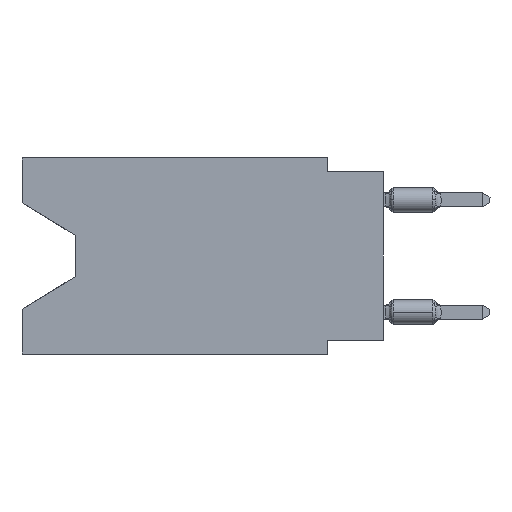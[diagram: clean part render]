
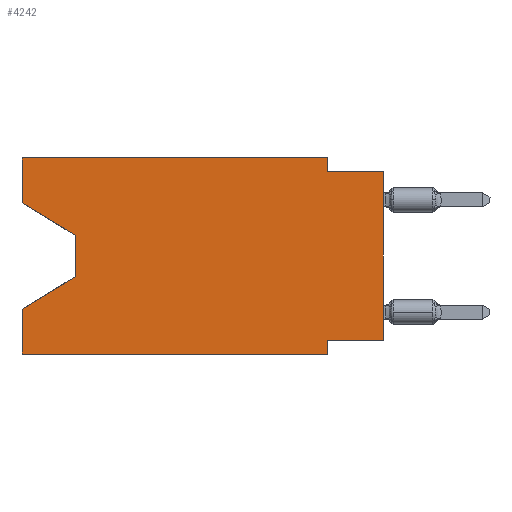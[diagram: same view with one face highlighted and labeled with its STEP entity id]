
A CAD part, left-side view. The second image highlights one B-rep face of the part: STEP entity #4242.
In plain terms, the highlighted planar face has unit normal (-1, 0, 0).
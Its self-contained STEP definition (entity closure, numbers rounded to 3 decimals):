
#185 = VECTOR ( 'NONE', #11894, 1000. ) ;
#356 = LINE ( 'NONE', #1703, #1404 ) ;
#411 = ORIENTED_EDGE ( 'NONE', *, *, #1171, .T. ) ;
#521 = CARTESIAN_POINT ( 'NONE',  ( 0., 16.383, -6.852 ) ) ;
#795 = ORIENTED_EDGE ( 'NONE', *, *, #1060, .F. ) ;
#810 = EDGE_CURVE ( 'NONE', #8249, #14332, #7333, .T. ) ;
#878 = DIRECTION ( 'NONE',  ( 0., 1., 0. ) ) ;
#1060 = EDGE_CURVE ( 'NONE', #10597, #8249, #9321, .T. ) ;
#1171 = EDGE_CURVE ( 'NONE', #6438, #5531, #4369, .T. ) ;
#1404 = VECTOR ( 'NONE', #15974, 1000. ) ;
#1484 = DIRECTION ( 'NONE',  ( 0., 0., 1. ) ) ;
#1649 = VECTOR ( 'NONE', #13506, 1000. ) ;
#1703 = CARTESIAN_POINT ( 'NONE',  ( 0., 16.383, 0. ) ) ;
#1808 = ORIENTED_EDGE ( 'NONE', *, *, #6206, .T. ) ;
#1897 = ORIENTED_EDGE ( 'NONE', *, *, #810, .F. ) ;
#1899 = EDGE_CURVE ( 'NONE', #4299, #14967, #3849, .T. ) ;
#2055 = DIRECTION ( 'NONE',  ( 0., 0., -1. ) ) ;
#2230 = ORIENTED_EDGE ( 'NONE', *, *, #13878, .F. ) ;
#2676 = CARTESIAN_POINT ( 'NONE',  ( 0., 0., 0. ) ) ;
#2705 = VECTOR ( 'NONE', #11100, 1000. ) ;
#2866 = DIRECTION ( 'NONE',  ( 0., -0.855, -0.519 ) ) ;
#3119 = DIRECTION ( 'NONE',  ( 0., 0.855, -0.519 ) ) ;
#3222 = LINE ( 'NONE', #3475, #2705 ) ;
#3268 = CARTESIAN_POINT ( 'NONE',  ( 0., 0., -0.635 ) ) ;
#3475 = CARTESIAN_POINT ( 'NONE',  ( 0., 13.97, -3.505 ) ) ;
#3585 = LINE ( 'NONE', #13564, #7026 ) ;
#3849 = LINE ( 'NONE', #15668, #185 ) ;
#4203 = CARTESIAN_POINT ( 'NONE',  ( 0., 16.383, -2.038 ) ) ;
#4235 = CARTESIAN_POINT ( 'NONE',  ( 0., 0., -0.635 ) ) ;
#4242 = ADVANCED_FACE ( 'NONE', ( #8076 ), #5472, .F. ) ;
#4299 = VERTEX_POINT ( 'NONE', #13042 ) ;
#4369 = LINE ( 'NONE', #12342, #7140 ) ;
#4659 = LINE ( 'NONE', #15152, #6732 ) ;
#4800 = EDGE_LOOP ( 'NONE', ( #8580, #10846, #411, #11090, #5326, #16095, #9362, #1808, #2230, #9218, #1897, #795 ) ) ;
#5311 = CARTESIAN_POINT ( 'NONE',  ( 0., 16.383, 0. ) ) ;
#5326 = ORIENTED_EDGE ( 'NONE', *, *, #11420, .T. ) ;
#5329 = CARTESIAN_POINT ( 'NONE',  ( 0., 16.383, -8.89 ) ) ;
#5387 = DIRECTION ( 'NONE',  ( 0., 0., 1. ) ) ;
#5408 = LINE ( 'NONE', #5329, #12397 ) ;
#5472 = PLANE ( 'NONE',  #11635 ) ;
#5508 = VERTEX_POINT ( 'NONE', #4235 ) ;
#5531 = VERTEX_POINT ( 'NONE', #521 ) ;
#5663 = EDGE_CURVE ( 'NONE', #11098, #6438, #3222, .T. ) ;
#6206 = EDGE_CURVE ( 'NONE', #13308, #5508, #6693, .T. ) ;
#6412 = EDGE_CURVE ( 'NONE', #13308, #4299, #4659, .T. ) ;
#6438 = VERTEX_POINT ( 'NONE', #13908 ) ;
#6693 = LINE ( 'NONE', #2676, #12910 ) ;
#6732 = VECTOR ( 'NONE', #878, 1000. ) ;
#6855 = VECTOR ( 'NONE', #9663, 1000. ) ;
#7026 = VECTOR ( 'NONE', #2055, 1000. ) ;
#7140 = VECTOR ( 'NONE', #3119, 1000. ) ;
#7333 = LINE ( 'NONE', #12450, #6855 ) ;
#7407 = VECTOR ( 'NONE', #2866, 1000. ) ;
#7524 = CARTESIAN_POINT ( 'NONE',  ( 0., 2.54, 0. ) ) ;
#8026 = CARTESIAN_POINT ( 'NONE',  ( 0., 13.97, -3.505 ) ) ;
#8076 = FACE_OUTER_BOUND ( 'NONE', #4800, .T. ) ;
#8249 = VERTEX_POINT ( 'NONE', #13566 ) ;
#8580 = ORIENTED_EDGE ( 'NONE', *, *, #10630, .T. ) ;
#9093 = DIRECTION ( 'NONE',  ( 0., 0., -1. ) ) ;
#9200 = VERTEX_POINT ( 'NONE', #12933 ) ;
#9218 = ORIENTED_EDGE ( 'NONE', *, *, #14282, .F. ) ;
#9241 = CARTESIAN_POINT ( 'NONE',  ( 0., 16.383, 0. ) ) ;
#9321 = LINE ( 'NONE', #5311, #15992 ) ;
#9362 = ORIENTED_EDGE ( 'NONE', *, *, #6412, .F. ) ;
#9394 = CARTESIAN_POINT ( 'NONE',  ( 0., 2.54, -8.89 ) ) ;
#9663 = DIRECTION ( 'NONE',  ( 0., -1., 0. ) ) ;
#10528 = DIRECTION ( 'NONE',  ( 0., -1., 0. ) ) ;
#10585 = DIRECTION ( 'NONE',  ( 1., 0., 0. ) ) ;
#10597 = VERTEX_POINT ( 'NONE', #13192 ) ;
#10630 = EDGE_CURVE ( 'NONE', #10597, #11098, #13033, .T. ) ;
#10755 = CARTESIAN_POINT ( 'NONE',  ( 0., 0., -8.255 ) ) ;
#10846 = ORIENTED_EDGE ( 'NONE', *, *, #5663, .T. ) ;
#11090 = ORIENTED_EDGE ( 'NONE', *, *, #11537, .F. ) ;
#11098 = VERTEX_POINT ( 'NONE', #8026 ) ;
#11100 = DIRECTION ( 'NONE',  ( 0., 0., -1. ) ) ;
#11236 = VERTEX_POINT ( 'NONE', #14808 ) ;
#11420 = EDGE_CURVE ( 'NONE', #11236, #14967, #5408, .T. ) ;
#11537 = EDGE_CURVE ( 'NONE', #11236, #5531, #356, .T. ) ;
#11635 = AXIS2_PLACEMENT_3D ( 'NONE', #9241, #10585, #9093 ) ;
#11894 = DIRECTION ( 'NONE',  ( 0., 0., -1. ) ) ;
#12325 = LINE ( 'NONE', #3268, #1649 ) ;
#12342 = CARTESIAN_POINT ( 'NONE',  ( 0., 13.97, -5.385 ) ) ;
#12397 = VECTOR ( 'NONE', #10528, 1000. ) ;
#12450 = CARTESIAN_POINT ( 'NONE',  ( 0., 16.383, 0. ) ) ;
#12910 = VECTOR ( 'NONE', #1484, 1000. ) ;
#12933 = CARTESIAN_POINT ( 'NONE',  ( 0., 2.54, -0.635 ) ) ;
#13033 = LINE ( 'NONE', #4203, #7407 ) ;
#13042 = CARTESIAN_POINT ( 'NONE',  ( 0., 2.54, -8.255 ) ) ;
#13192 = CARTESIAN_POINT ( 'NONE',  ( 0., 16.383, -2.038 ) ) ;
#13308 = VERTEX_POINT ( 'NONE', #10755 ) ;
#13506 = DIRECTION ( 'NONE',  ( 0., -1., 0. ) ) ;
#13564 = CARTESIAN_POINT ( 'NONE',  ( 0., 2.54, 0. ) ) ;
#13566 = CARTESIAN_POINT ( 'NONE',  ( 0., 16.383, 0. ) ) ;
#13878 = EDGE_CURVE ( 'NONE', #9200, #5508, #12325, .T. ) ;
#13908 = CARTESIAN_POINT ( 'NONE',  ( 0., 13.97, -5.385 ) ) ;
#14282 = EDGE_CURVE ( 'NONE', #14332, #9200, #3585, .T. ) ;
#14332 = VERTEX_POINT ( 'NONE', #7524 ) ;
#14808 = CARTESIAN_POINT ( 'NONE',  ( 0., 16.383, -8.89 ) ) ;
#14967 = VERTEX_POINT ( 'NONE', #9394 ) ;
#15152 = CARTESIAN_POINT ( 'NONE',  ( 0., 0., -8.255 ) ) ;
#15668 = CARTESIAN_POINT ( 'NONE',  ( 0., 2.54, -8.89 ) ) ;
#15974 = DIRECTION ( 'NONE',  ( 0., 0., 1. ) ) ;
#15992 = VECTOR ( 'NONE', #5387, 1000. ) ;
#16095 = ORIENTED_EDGE ( 'NONE', *, *, #1899, .F. ) ;
